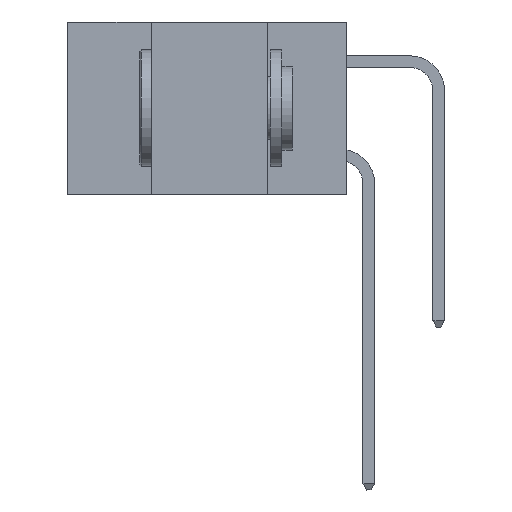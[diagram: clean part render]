
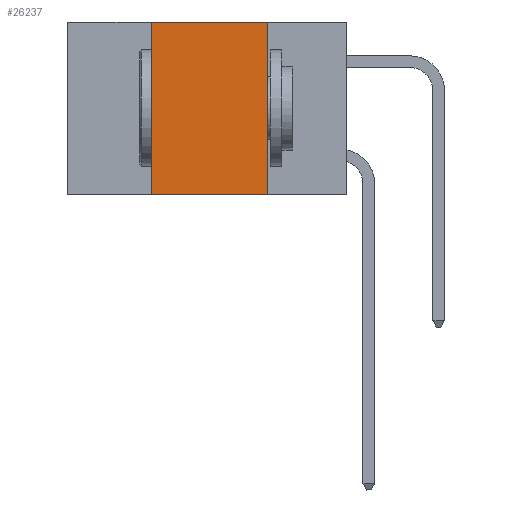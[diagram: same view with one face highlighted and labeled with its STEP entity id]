
A CAD part, left-side view. The second image highlights one B-rep face of the part: STEP entity #26237.
In plain terms, the highlighted planar face has unit normal (-1, 0, 0).
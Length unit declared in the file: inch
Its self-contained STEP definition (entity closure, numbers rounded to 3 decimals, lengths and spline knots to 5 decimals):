
#349 = LINE ( 'NONE', #6147, #13888 ) ;
#722 = VECTOR ( 'NONE', #35455, 39.37008 ) ;
#2764 = PLANE ( 'NONE',  #17277 ) ;
#2859 = EDGE_CURVE ( 'NONE', #20473, #27855, #349, .T. ) ;
#2888 = DIRECTION ( 'NONE',  ( 1., 0., 0. ) ) ;
#5067 = LINE ( 'NONE', #18492, #33788 ) ;
#6147 = CARTESIAN_POINT ( 'NONE',  ( 0., 0.6, -0.37 ) ) ;
#7752 = LINE ( 'NONE', #33919, #722 ) ;
#9317 = ORIENTED_EDGE ( 'NONE', *, *, #23199, .F. ) ;
#10711 = DIRECTION ( 'NONE',  ( 0., 0., 1. ) ) ;
#13753 = EDGE_CURVE ( 'NONE', #14102, #26787, #7752, .T. ) ;
#13888 = VECTOR ( 'NONE', #19951, 39.37008 ) ;
#14044 = DIRECTION ( 'NONE',  ( 0., 0., -1. ) ) ;
#14102 = VERTEX_POINT ( 'NONE', #26381 ) ;
#15056 = CARTESIAN_POINT ( 'NONE',  ( 0., 0.17, 0. ) ) ;
#17277 = AXIS2_PLACEMENT_3D ( 'NONE', #28063, #2888, #14044 ) ;
#18492 = CARTESIAN_POINT ( 'NONE',  ( 0., 0.17, 0. ) ) ;
#19951 = DIRECTION ( 'NONE',  ( 0., -1., 0. ) ) ;
#20473 = VERTEX_POINT ( 'NONE', #27796 ) ;
#22983 = FACE_OUTER_BOUND ( 'NONE', #27384, .T. ) ;
#23199 = EDGE_CURVE ( 'NONE', #20473, #14102, #23815, .T. ) ;
#23815 = LINE ( 'NONE', #32719, #33418 ) ;
#25122 = ORIENTED_EDGE ( 'NONE', *, *, #13753, .F. ) ;
#26237 = ADVANCED_FACE ( 'NONE', ( #22983 ), #2764, .F. ) ;
#26381 = CARTESIAN_POINT ( 'NONE',  ( 0., 0.42, 0. ) ) ;
#26787 = VERTEX_POINT ( 'NONE', #15056 ) ;
#27384 = EDGE_LOOP ( 'NONE', ( #28249, #25122, #9317, #35317 ) ) ;
#27796 = CARTESIAN_POINT ( 'NONE',  ( 0., 0.42, -0.37 ) ) ;
#27855 = VERTEX_POINT ( 'NONE', #33785 ) ;
#28063 = CARTESIAN_POINT ( 'NONE',  ( 0., 0.6, 0. ) ) ;
#28249 = ORIENTED_EDGE ( 'NONE', *, *, #28274, .F. ) ;
#28274 = EDGE_CURVE ( 'NONE', #26787, #27855, #5067, .T. ) ;
#29383 = DIRECTION ( 'NONE',  ( 0., 0., -1. ) ) ;
#32719 = CARTESIAN_POINT ( 'NONE',  ( 0., 0.42, 0. ) ) ;
#33418 = VECTOR ( 'NONE', #10711, 39.37008 ) ;
#33785 = CARTESIAN_POINT ( 'NONE',  ( 0., 0.17, -0.37 ) ) ;
#33788 = VECTOR ( 'NONE', #29383, 39.37008 ) ;
#33919 = CARTESIAN_POINT ( 'NONE',  ( 0., 0.6, 0. ) ) ;
#35317 = ORIENTED_EDGE ( 'NONE', *, *, #2859, .T. ) ;
#35455 = DIRECTION ( 'NONE',  ( 0., -1., 0. ) ) ;
